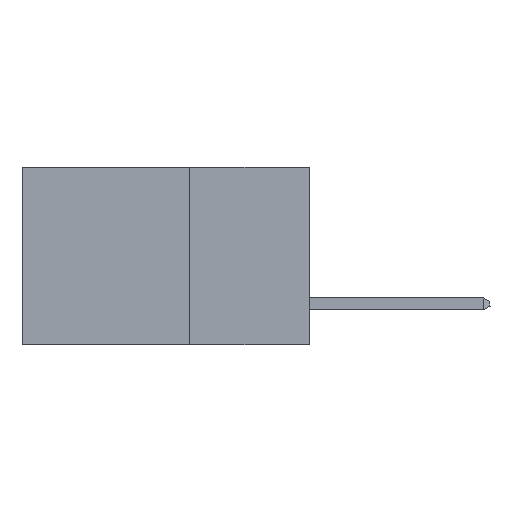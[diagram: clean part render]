
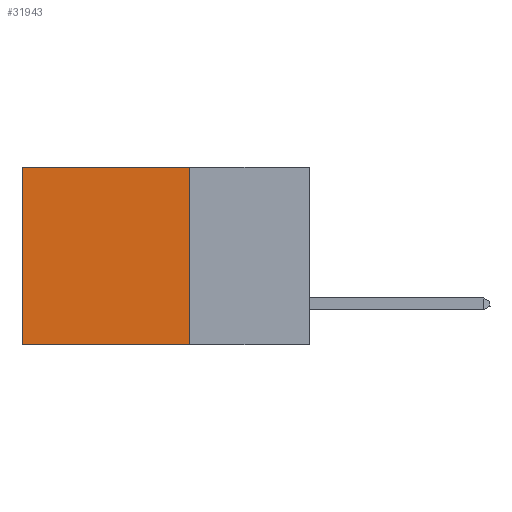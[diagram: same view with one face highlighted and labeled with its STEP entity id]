
A CAD part, left-side view. The second image highlights one B-rep face of the part: STEP entity #31943.
In plain terms, the highlighted planar face has unit normal (-1, 0, 0).
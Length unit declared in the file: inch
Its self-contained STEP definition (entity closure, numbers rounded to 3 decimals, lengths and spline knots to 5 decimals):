
#1149 = CARTESIAN_POINT ( 'NONE',  ( 0.2875, 0.25, 0. ) ) ;
#1717 = VERTEX_POINT ( 'NONE', #27165 ) ;
#3492 = DIRECTION ( 'NONE',  ( 0., 1., 0. ) ) ;
#4532 = VERTEX_POINT ( 'NONE', #13609 ) ;
#4546 = PLANE ( 'NONE',  #22933 ) ;
#5115 = ORIENTED_EDGE ( 'NONE', *, *, #11260, .T. ) ;
#5156 = EDGE_LOOP ( 'NONE', ( #29121, #32793, #31781, #5115 ) ) ;
#5204 = LINE ( 'NONE', #1149, #20830 ) ;
#5602 = DIRECTION ( 'NONE',  ( 0., 0., -1. ) ) ;
#8492 = EDGE_CURVE ( 'NONE', #1717, #15517, #9415, .T. ) ;
#9415 = LINE ( 'NONE', #19070, #22940 ) ;
#10141 = CARTESIAN_POINT ( 'NONE',  ( 0.2875, 0.25, 0. ) ) ;
#10281 = VERTEX_POINT ( 'NONE', #10141 ) ;
#11260 = EDGE_CURVE ( 'NONE', #10281, #1717, #11271, .T. ) ;
#11271 = LINE ( 'NONE', #19280, #26057 ) ;
#11330 = EDGE_CURVE ( 'NONE', #4532, #15517, #26853, .T. ) ;
#11474 = FACE_OUTER_BOUND ( 'NONE', #5156, .T. ) ;
#13609 = CARTESIAN_POINT ( 'NONE',  ( 0.2875, 0.25, -0.37 ) ) ;
#15022 = CARTESIAN_POINT ( 'NONE',  ( 0.2875, 0.25, 0. ) ) ;
#15517 = VERTEX_POINT ( 'NONE', #32735 ) ;
#16472 = DIRECTION ( 'NONE',  ( 0., 0., -1. ) ) ;
#16980 = DIRECTION ( 'NONE',  ( 0., 1., 0. ) ) ;
#19070 = CARTESIAN_POINT ( 'NONE',  ( 0.2875, 0.6, 0. ) ) ;
#19280 = CARTESIAN_POINT ( 'NONE',  ( 0.2875, 0.25, 0. ) ) ;
#20830 = VECTOR ( 'NONE', #16472, 39.37008 ) ;
#22933 = AXIS2_PLACEMENT_3D ( 'NONE', #15022, #30605, #32921 ) ;
#22940 = VECTOR ( 'NONE', #5602, 39.37008 ) ;
#23146 = VECTOR ( 'NONE', #16980, 39.37008 ) ;
#26057 = VECTOR ( 'NONE', #3492, 39.37008 ) ;
#26853 = LINE ( 'NONE', #30152, #23146 ) ;
#27165 = CARTESIAN_POINT ( 'NONE',  ( 0.2875, 0.6, 0. ) ) ;
#29121 = ORIENTED_EDGE ( 'NONE', *, *, #8492, .T. ) ;
#30152 = CARTESIAN_POINT ( 'NONE',  ( 0.2875, 0.25, -0.37 ) ) ;
#30206 = EDGE_CURVE ( 'NONE', #10281, #4532, #5204, .T. ) ;
#30605 = DIRECTION ( 'NONE',  ( 1., 0., 0. ) ) ;
#31781 = ORIENTED_EDGE ( 'NONE', *, *, #30206, .F. ) ;
#31943 = ADVANCED_FACE ( 'NONE', ( #11474 ), #4546, .F. ) ;
#32735 = CARTESIAN_POINT ( 'NONE',  ( 0.2875, 0.6, -0.37 ) ) ;
#32793 = ORIENTED_EDGE ( 'NONE', *, *, #11330, .F. ) ;
#32921 = DIRECTION ( 'NONE',  ( 0., 0., -1. ) ) ;
